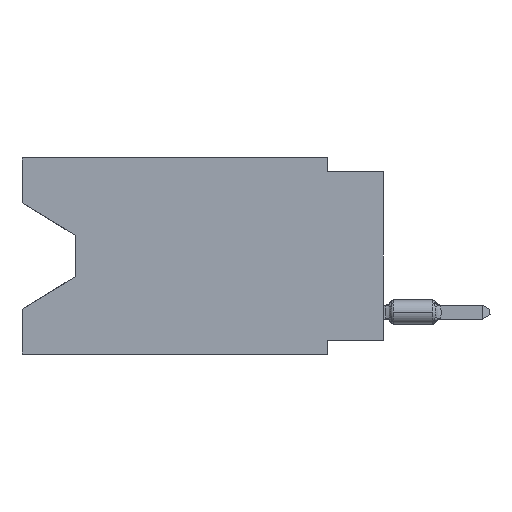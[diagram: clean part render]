
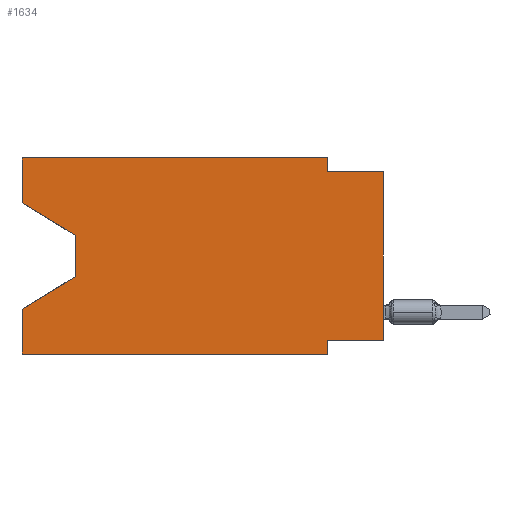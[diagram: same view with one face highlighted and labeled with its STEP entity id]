
A CAD part, left-side view. The second image highlights one B-rep face of the part: STEP entity #1634.
In plain terms, the highlighted planar face has unit normal (-1, 0, 0).
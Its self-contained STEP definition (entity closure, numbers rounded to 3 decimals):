
#5 = VECTOR ( 'NONE', #7616, 1000. ) ;
#276 = LINE ( 'NONE', #9998, #11186 ) ;
#592 = DIRECTION ( 'NONE',  ( 0., -1., 0. ) ) ;
#756 = CARTESIAN_POINT ( 'NONE',  ( 0., 0., -8.255 ) ) ;
#1081 = EDGE_CURVE ( 'NONE', #31130, #17988, #11241, .T. ) ;
#1092 = ORIENTED_EDGE ( 'NONE', *, *, #14705, .F. ) ;
#1437 = LINE ( 'NONE', #25823, #15412 ) ;
#1465 = ORIENTED_EDGE ( 'NONE', *, *, #29700, .T. ) ;
#1634 = ADVANCED_FACE ( 'NONE', ( #22389 ), #8203, .F. ) ;
#1697 = DIRECTION ( 'NONE',  ( 0., -1., 0. ) ) ;
#1709 = ORIENTED_EDGE ( 'NONE', *, *, #18261, .T. ) ;
#2175 = ORIENTED_EDGE ( 'NONE', *, *, #1081, .F. ) ;
#2472 = AXIS2_PLACEMENT_3D ( 'NONE', #3726, #10424, #27940 ) ;
#2484 = ORIENTED_EDGE ( 'NONE', *, *, #3792, .T. ) ;
#3017 = VERTEX_POINT ( 'NONE', #9439 ) ;
#3105 = VECTOR ( 'NONE', #4662, 1000. ) ;
#3240 = ORIENTED_EDGE ( 'NONE', *, *, #21709, .T. ) ;
#3595 = DIRECTION ( 'NONE',  ( 0., 1., 0. ) ) ;
#3726 = CARTESIAN_POINT ( 'NONE',  ( 0., 16.383, 0. ) ) ;
#3792 = EDGE_CURVE ( 'NONE', #13963, #30853, #30367, .T. ) ;
#4274 = ORIENTED_EDGE ( 'NONE', *, *, #13928, .F. ) ;
#4662 = DIRECTION ( 'NONE',  ( 0., 0., 1. ) ) ;
#4804 = CARTESIAN_POINT ( 'NONE',  ( 0., 13.97, -3.505 ) ) ;
#4810 = EDGE_CURVE ( 'NONE', #3017, #8985, #13166, .T. ) ;
#6430 = ORIENTED_EDGE ( 'NONE', *, *, #25531, .F. ) ;
#6602 = CARTESIAN_POINT ( 'NONE',  ( 0., 0., -8.255 ) ) ;
#6689 = VERTEX_POINT ( 'NONE', #27486 ) ;
#7616 = DIRECTION ( 'NONE',  ( 0., 0., 1. ) ) ;
#8170 = VERTEX_POINT ( 'NONE', #11365 ) ;
#8203 = PLANE ( 'NONE',  #2472 ) ;
#8985 = VERTEX_POINT ( 'NONE', #12129 ) ;
#9184 = VERTEX_POINT ( 'NONE', #20082 ) ;
#9214 = VERTEX_POINT ( 'NONE', #10367 ) ;
#9254 = CARTESIAN_POINT ( 'NONE',  ( 0., 2.54, 0. ) ) ;
#9439 = CARTESIAN_POINT ( 'NONE',  ( 0., 16.383, 0. ) ) ;
#9682 = VECTOR ( 'NONE', #1697, 1000. ) ;
#9705 = LINE ( 'NONE', #14618, #5 ) ;
#9756 = CARTESIAN_POINT ( 'NONE',  ( 0., 16.383, 0. ) ) ;
#9998 = CARTESIAN_POINT ( 'NONE',  ( 0., 0., -0.635 ) ) ;
#10203 = EDGE_CURVE ( 'NONE', #9184, #19553, #18554, .T. ) ;
#10220 = DIRECTION ( 'NONE',  ( 0., 0., -1. ) ) ;
#10367 = CARTESIAN_POINT ( 'NONE',  ( 0., 2.54, -8.89 ) ) ;
#10424 = DIRECTION ( 'NONE',  ( 1., 0., 0. ) ) ;
#10519 = VECTOR ( 'NONE', #23919, 1000. ) ;
#11084 = CARTESIAN_POINT ( 'NONE',  ( 0., 16.383, -2.038 ) ) ;
#11186 = VECTOR ( 'NONE', #29913, 1000. ) ;
#11234 = DIRECTION ( 'NONE',  ( 0., 0., 1. ) ) ;
#11241 = LINE ( 'NONE', #6602, #21799 ) ;
#11270 = CARTESIAN_POINT ( 'NONE',  ( 0., 16.383, -8.89 ) ) ;
#11334 = DIRECTION ( 'NONE',  ( 0., 0.855, -0.519 ) ) ;
#11365 = CARTESIAN_POINT ( 'NONE',  ( 0., 2.54, -0.635 ) ) ;
#11596 = ORIENTED_EDGE ( 'NONE', *, *, #30672, .F. ) ;
#11633 = LINE ( 'NONE', #9254, #10519 ) ;
#11660 = VECTOR ( 'NONE', #10220, 1000. ) ;
#12129 = CARTESIAN_POINT ( 'NONE',  ( 0., 2.54, 0. ) ) ;
#12316 = CARTESIAN_POINT ( 'NONE',  ( 0., 2.54, -8.255 ) ) ;
#13166 = LINE ( 'NONE', #17337, #17351 ) ;
#13638 = ORIENTED_EDGE ( 'NONE', *, *, #4810, .F. ) ;
#13928 = EDGE_CURVE ( 'NONE', #17988, #9214, #19534, .T. ) ;
#13963 = VERTEX_POINT ( 'NONE', #27179 ) ;
#14618 = CARTESIAN_POINT ( 'NONE',  ( 0., 0., 0. ) ) ;
#14705 = EDGE_CURVE ( 'NONE', #8170, #29183, #276, .T. ) ;
#15036 = CARTESIAN_POINT ( 'NONE',  ( 0., 2.54, -8.89 ) ) ;
#15206 = VECTOR ( 'NONE', #20515, 1000. ) ;
#15412 = VECTOR ( 'NONE', #11334, 1000. ) ;
#15932 = CARTESIAN_POINT ( 'NONE',  ( 0., 13.97, -3.505 ) ) ;
#16150 = CARTESIAN_POINT ( 'NONE',  ( 0., 16.383, 0. ) ) ;
#16153 = EDGE_LOOP ( 'NONE', ( #2484, #3240, #1709, #23395, #22588, #4274, #2175, #1465, #1092, #6430, #13638, #11596 ) ) ;
#17215 = LINE ( 'NONE', #4804, #11660 ) ;
#17337 = CARTESIAN_POINT ( 'NONE',  ( 0., 16.383, 0. ) ) ;
#17351 = VECTOR ( 'NONE', #592, 1000. ) ;
#17988 = VERTEX_POINT ( 'NONE', #12316 ) ;
#18261 = EDGE_CURVE ( 'NONE', #6689, #19553, #1437, .T. ) ;
#18554 = LINE ( 'NONE', #16150, #27376 ) ;
#19534 = LINE ( 'NONE', #15036, #30084 ) ;
#19553 = VERTEX_POINT ( 'NONE', #21771 ) ;
#20082 = CARTESIAN_POINT ( 'NONE',  ( 0., 16.383, -8.89 ) ) ;
#20515 = DIRECTION ( 'NONE',  ( 0., -0.855, -0.519 ) ) ;
#20589 = CARTESIAN_POINT ( 'NONE',  ( 0., 0., -0.635 ) ) ;
#21561 = LINE ( 'NONE', #9756, #3105 ) ;
#21709 = EDGE_CURVE ( 'NONE', #30853, #6689, #17215, .T. ) ;
#21771 = CARTESIAN_POINT ( 'NONE',  ( 0., 16.383, -6.852 ) ) ;
#21799 = VECTOR ( 'NONE', #3595, 1000. ) ;
#22389 = FACE_OUTER_BOUND ( 'NONE', #16153, .T. ) ;
#22588 = ORIENTED_EDGE ( 'NONE', *, *, #30028, .T. ) ;
#23395 = ORIENTED_EDGE ( 'NONE', *, *, #10203, .F. ) ;
#23919 = DIRECTION ( 'NONE',  ( 0., 0., -1. ) ) ;
#25531 = EDGE_CURVE ( 'NONE', #8985, #8170, #11633, .T. ) ;
#25823 = CARTESIAN_POINT ( 'NONE',  ( 0., 13.97, -5.385 ) ) ;
#27179 = CARTESIAN_POINT ( 'NONE',  ( 0., 16.383, -2.038 ) ) ;
#27376 = VECTOR ( 'NONE', #11234, 1000. ) ;
#27486 = CARTESIAN_POINT ( 'NONE',  ( 0., 13.97, -5.385 ) ) ;
#27940 = DIRECTION ( 'NONE',  ( 0., 0., -1. ) ) ;
#29183 = VERTEX_POINT ( 'NONE', #20589 ) ;
#29396 = DIRECTION ( 'NONE',  ( 0., 0., -1. ) ) ;
#29700 = EDGE_CURVE ( 'NONE', #31130, #29183, #9705, .T. ) ;
#29913 = DIRECTION ( 'NONE',  ( 0., -1., 0. ) ) ;
#30028 = EDGE_CURVE ( 'NONE', #9184, #9214, #30549, .T. ) ;
#30084 = VECTOR ( 'NONE', #29396, 1000. ) ;
#30367 = LINE ( 'NONE', #11084, #15206 ) ;
#30549 = LINE ( 'NONE', #11270, #9682 ) ;
#30672 = EDGE_CURVE ( 'NONE', #13963, #3017, #21561, .T. ) ;
#30853 = VERTEX_POINT ( 'NONE', #15932 ) ;
#31130 = VERTEX_POINT ( 'NONE', #756 ) ;
